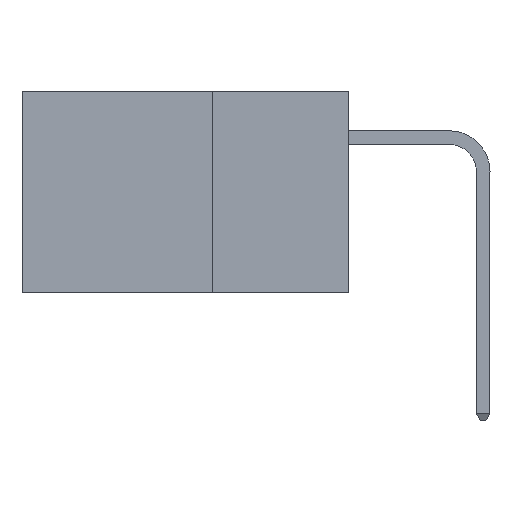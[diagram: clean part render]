
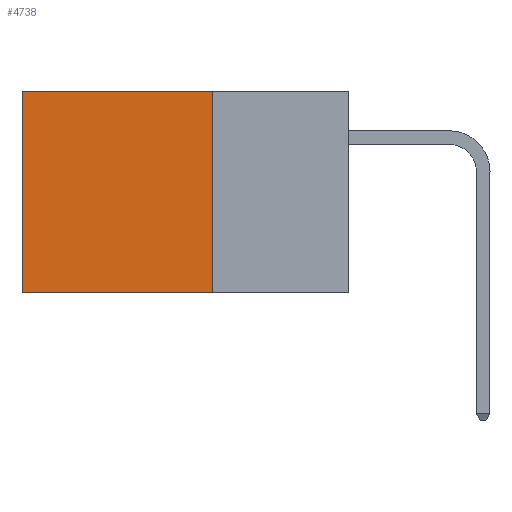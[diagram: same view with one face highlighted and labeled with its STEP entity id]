
A CAD part, left-side view. The second image highlights one B-rep face of the part: STEP entity #4738.
In plain terms, the highlighted planar face has unit normal (-1, 0, 0).
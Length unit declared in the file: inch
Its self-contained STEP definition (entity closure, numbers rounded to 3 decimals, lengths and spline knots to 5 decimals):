
#213 = DIRECTION ( 'NONE',  ( 0., 1., 0. ) ) ;
#466 = EDGE_CURVE ( 'NONE', #1810, #9491, #1905, .T. ) ;
#619 = LINE ( 'NONE', #12471, #928 ) ;
#867 = ORIENTED_EDGE ( 'NONE', *, *, #7588, .F. ) ;
#928 = VECTOR ( 'NONE', #12392, 39.37008 ) ;
#1810 = VERTEX_POINT ( 'NONE', #10217 ) ;
#1905 = LINE ( 'NONE', #2539, #11760 ) ;
#2197 = LINE ( 'NONE', #6033, #5545 ) ;
#2232 = VERTEX_POINT ( 'NONE', #11996 ) ;
#2286 = DIRECTION ( 'NONE',  ( 1., 0., 0. ) ) ;
#2539 = CARTESIAN_POINT ( 'NONE',  ( 0.2875, 0.6, 0. ) ) ;
#3084 = CARTESIAN_POINT ( 'NONE',  ( 0.2875, 0.25, -0.37 ) ) ;
#3153 = LINE ( 'NONE', #8071, #12552 ) ;
#3293 = EDGE_CURVE ( 'NONE', #2232, #1810, #2197, .T. ) ;
#3572 = ORIENTED_EDGE ( 'NONE', *, *, #6324, .F. ) ;
#3884 = ORIENTED_EDGE ( 'NONE', *, *, #3293, .T. ) ;
#4086 = DIRECTION ( 'NONE',  ( 0., 1., 0. ) ) ;
#4308 = DIRECTION ( 'NONE',  ( 0., 0., -1. ) ) ;
#4462 = AXIS2_PLACEMENT_3D ( 'NONE', #9070, #2286, #4308 ) ;
#4738 = ADVANCED_FACE ( 'NONE', ( #10351 ), #9194, .F. ) ;
#4786 = CARTESIAN_POINT ( 'NONE',  ( 0.2875, 0.6, -0.37 ) ) ;
#5257 = ORIENTED_EDGE ( 'NONE', *, *, #466, .T. ) ;
#5545 = VECTOR ( 'NONE', #4086, 39.37008 ) ;
#6033 = CARTESIAN_POINT ( 'NONE',  ( 0.2875, 0.25, 0. ) ) ;
#6324 = EDGE_CURVE ( 'NONE', #2232, #12035, #619, .T. ) ;
#7588 = EDGE_CURVE ( 'NONE', #12035, #9491, #3153, .T. ) ;
#8071 = CARTESIAN_POINT ( 'NONE',  ( 0.2875, 0.25, -0.37 ) ) ;
#8342 = DIRECTION ( 'NONE',  ( 0., 0., -1. ) ) ;
#9070 = CARTESIAN_POINT ( 'NONE',  ( 0.2875, 0.25, 0. ) ) ;
#9194 = PLANE ( 'NONE',  #4462 ) ;
#9491 = VERTEX_POINT ( 'NONE', #4786 ) ;
#10217 = CARTESIAN_POINT ( 'NONE',  ( 0.2875, 0.6, 0. ) ) ;
#10351 = FACE_OUTER_BOUND ( 'NONE', #12324, .T. ) ;
#11760 = VECTOR ( 'NONE', #8342, 39.37008 ) ;
#11996 = CARTESIAN_POINT ( 'NONE',  ( 0.2875, 0.25, 0. ) ) ;
#12035 = VERTEX_POINT ( 'NONE', #3084 ) ;
#12324 = EDGE_LOOP ( 'NONE', ( #5257, #867, #3572, #3884 ) ) ;
#12392 = DIRECTION ( 'NONE',  ( 0., 0., -1. ) ) ;
#12471 = CARTESIAN_POINT ( 'NONE',  ( 0.2875, 0.25, 0. ) ) ;
#12552 = VECTOR ( 'NONE', #213, 39.37008 ) ;
